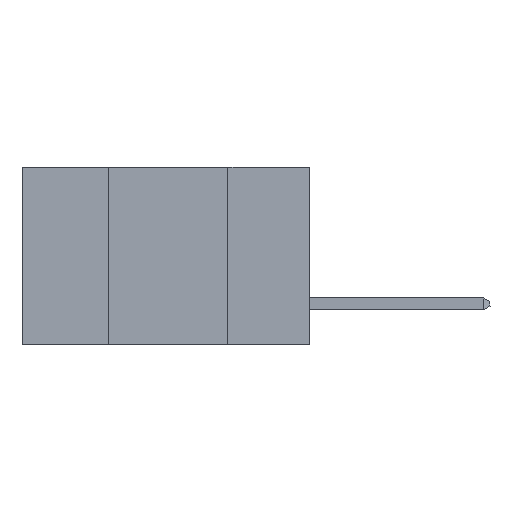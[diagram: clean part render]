
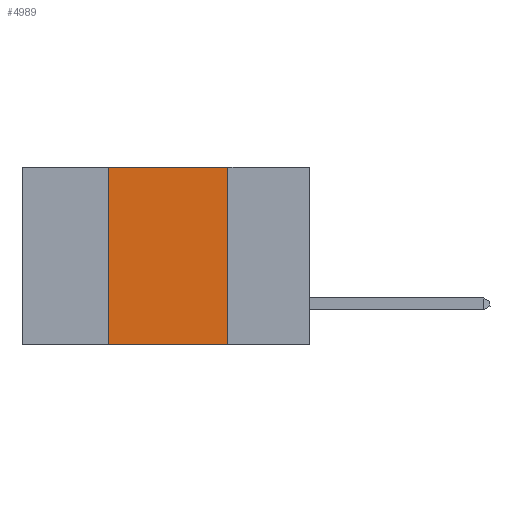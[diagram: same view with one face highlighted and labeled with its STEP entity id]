
A CAD part, left-side view. The second image highlights one B-rep face of the part: STEP entity #4989.
In plain terms, the highlighted planar face has unit normal (-1, 0, 0).
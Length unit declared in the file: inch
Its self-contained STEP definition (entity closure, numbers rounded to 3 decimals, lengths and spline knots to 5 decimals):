
#733 = CARTESIAN_POINT ( 'NONE',  ( 0., 0.17, -0.37 ) ) ;
#886 = LINE ( 'NONE', #8748, #9145 ) ;
#2779 = CARTESIAN_POINT ( 'NONE',  ( 0., 0.42, -0.37 ) ) ;
#4153 = ORIENTED_EDGE ( 'NONE', *, *, #6788, .F. ) ;
#4176 = EDGE_LOOP ( 'NONE', ( #20481, #8011, #4153, #8527 ) ) ;
#4989 = ADVANCED_FACE ( 'NONE', ( #13998 ), #8063, .F. ) ;
#5245 = VECTOR ( 'NONE', #11498, 39.37008 ) ;
#6757 = VERTEX_POINT ( 'NONE', #12754 ) ;
#6788 = EDGE_CURVE ( 'NONE', #14500, #21047, #17710, .T. ) ;
#6821 = EDGE_CURVE ( 'NONE', #21047, #6757, #16703, .T. ) ;
#7862 = DIRECTION ( 'NONE',  ( 0., 0., 1. ) ) ;
#7987 = VECTOR ( 'NONE', #11257, 39.37008 ) ;
#8011 = ORIENTED_EDGE ( 'NONE', *, *, #6821, .F. ) ;
#8063 = PLANE ( 'NONE',  #17522 ) ;
#8527 = ORIENTED_EDGE ( 'NONE', *, *, #15577, .T. ) ;
#8748 = CARTESIAN_POINT ( 'NONE',  ( 0., 0.6, -0.37 ) ) ;
#9145 = VECTOR ( 'NONE', #10423, 39.37008 ) ;
#9512 = CARTESIAN_POINT ( 'NONE',  ( 0., 0.42, 0. ) ) ;
#9726 = DIRECTION ( 'NONE',  ( 1., 0., 0. ) ) ;
#9833 = VERTEX_POINT ( 'NONE', #733 ) ;
#10423 = DIRECTION ( 'NONE',  ( 0., -1., 0. ) ) ;
#10663 = LINE ( 'NONE', #13462, #5245 ) ;
#10808 = EDGE_CURVE ( 'NONE', #6757, #9833, #10663, .T. ) ;
#11257 = DIRECTION ( 'NONE',  ( 0., -1., 0. ) ) ;
#11498 = DIRECTION ( 'NONE',  ( 0., 0., -1. ) ) ;
#12499 = CARTESIAN_POINT ( 'NONE',  ( 0., 0.42, 0. ) ) ;
#12754 = CARTESIAN_POINT ( 'NONE',  ( 0., 0.17, 0. ) ) ;
#13462 = CARTESIAN_POINT ( 'NONE',  ( 0., 0.17, 0. ) ) ;
#13998 = FACE_OUTER_BOUND ( 'NONE', #4176, .T. ) ;
#14500 = VERTEX_POINT ( 'NONE', #2779 ) ;
#15577 = EDGE_CURVE ( 'NONE', #14500, #9833, #886, .T. ) ;
#16703 = LINE ( 'NONE', #19344, #7987 ) ;
#17204 = VECTOR ( 'NONE', #7862, 39.37008 ) ;
#17522 = AXIS2_PLACEMENT_3D ( 'NONE', #17792, #9726, #21056 ) ;
#17710 = LINE ( 'NONE', #9512, #17204 ) ;
#17792 = CARTESIAN_POINT ( 'NONE',  ( 0., 0.6, 0. ) ) ;
#19344 = CARTESIAN_POINT ( 'NONE',  ( 0., 0.6, 0. ) ) ;
#20481 = ORIENTED_EDGE ( 'NONE', *, *, #10808, .F. ) ;
#21047 = VERTEX_POINT ( 'NONE', #12499 ) ;
#21056 = DIRECTION ( 'NONE',  ( 0., 0., -1. ) ) ;
